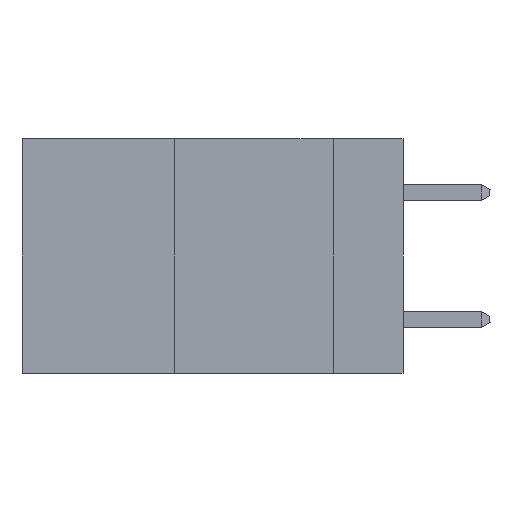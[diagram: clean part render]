
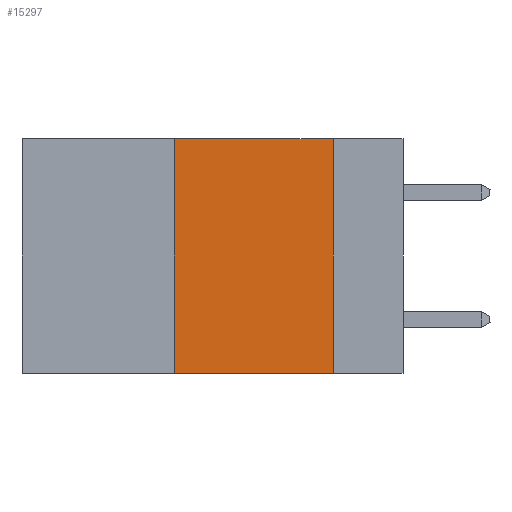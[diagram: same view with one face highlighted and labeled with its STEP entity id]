
A CAD part, left-side view. The second image highlights one B-rep face of the part: STEP entity #15297.
In plain terms, the highlighted planar face has unit normal (-1, 0, 0).
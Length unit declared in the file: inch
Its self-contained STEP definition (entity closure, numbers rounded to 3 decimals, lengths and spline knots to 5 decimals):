
#25 = LINE ( 'NONE', #27229, #5621 ) ;
#648 = DIRECTION ( 'NONE',  ( 0., 0., -1. ) ) ;
#1233 = DIRECTION ( 'NONE',  ( 0., 0., -1. ) ) ;
#2439 = DIRECTION ( 'NONE',  ( 0., -1., 0. ) ) ;
#3744 = PLANE ( 'NONE',  #6791 ) ;
#5017 = FACE_OUTER_BOUND ( 'NONE', #23968, .T. ) ;
#5234 = VERTEX_POINT ( 'NONE', #12686 ) ;
#5621 = VECTOR ( 'NONE', #29602, 39.37008 ) ;
#5787 = VECTOR ( 'NONE', #2439, 39.37008 ) ;
#6271 = LINE ( 'NONE', #24755, #24053 ) ;
#6791 = AXIS2_PLACEMENT_3D ( 'NONE', #15435, #15531, #1233 ) ;
#7884 = EDGE_CURVE ( 'NONE', #27666, #5234, #8715, .T. ) ;
#8212 = DIRECTION ( 'NONE',  ( 0., -1., 0. ) ) ;
#8715 = LINE ( 'NONE', #9591, #5787 ) ;
#9356 = ORIENTED_EDGE ( 'NONE', *, *, #28374, .F. ) ;
#9591 = CARTESIAN_POINT ( 'NONE',  ( 0., 0.6, -0.37 ) ) ;
#10517 = CARTESIAN_POINT ( 'NONE',  ( 0., 0.36, 0. ) ) ;
#12686 = CARTESIAN_POINT ( 'NONE',  ( 0., 0.11, -0.37 ) ) ;
#13634 = VECTOR ( 'NONE', #648, 39.37008 ) ;
#15297 = ADVANCED_FACE ( 'NONE', ( #5017 ), #3744, .F. ) ;
#15435 = CARTESIAN_POINT ( 'NONE',  ( 0., 0.6, 0. ) ) ;
#15466 = ORIENTED_EDGE ( 'NONE', *, *, #19849, .F. ) ;
#15531 = DIRECTION ( 'NONE',  ( 1., 0., 0. ) ) ;
#17394 = EDGE_CURVE ( 'NONE', #27666, #17403, #25, .T. ) ;
#17403 = VERTEX_POINT ( 'NONE', #10517 ) ;
#19849 = EDGE_CURVE ( 'NONE', #29978, #5234, #23837, .T. ) ;
#20090 = CARTESIAN_POINT ( 'NONE',  ( 0., 0.36, -0.37 ) ) ;
#22358 = CARTESIAN_POINT ( 'NONE',  ( 0., 0.11, 0. ) ) ;
#22822 = ORIENTED_EDGE ( 'NONE', *, *, #7884, .T. ) ;
#23837 = LINE ( 'NONE', #30484, #13634 ) ;
#23968 = EDGE_LOOP ( 'NONE', ( #15466, #9356, #29020, #22822 ) ) ;
#24053 = VECTOR ( 'NONE', #8212, 39.37008 ) ;
#24755 = CARTESIAN_POINT ( 'NONE',  ( 0., 0.6, 0. ) ) ;
#27229 = CARTESIAN_POINT ( 'NONE',  ( 0., 0.36, 0. ) ) ;
#27666 = VERTEX_POINT ( 'NONE', #20090 ) ;
#28374 = EDGE_CURVE ( 'NONE', #17403, #29978, #6271, .T. ) ;
#29020 = ORIENTED_EDGE ( 'NONE', *, *, #17394, .F. ) ;
#29602 = DIRECTION ( 'NONE',  ( 0., 0., 1. ) ) ;
#29978 = VERTEX_POINT ( 'NONE', #22358 ) ;
#30484 = CARTESIAN_POINT ( 'NONE',  ( 0., 0.11, 0. ) ) ;
